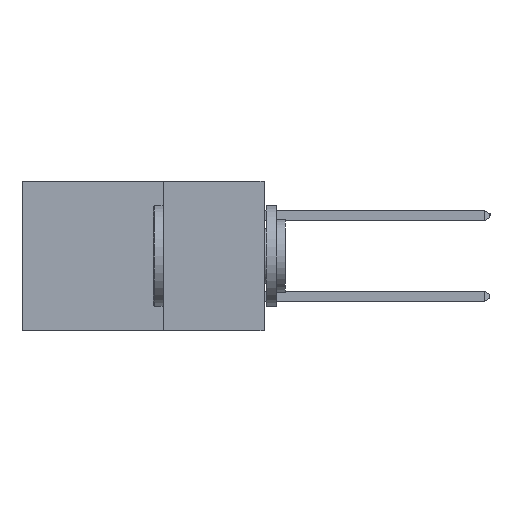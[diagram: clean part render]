
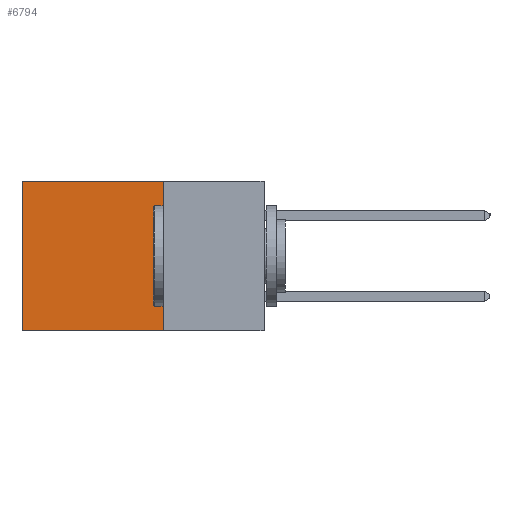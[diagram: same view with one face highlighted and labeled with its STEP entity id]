
A CAD part, left-side view. The second image highlights one B-rep face of the part: STEP entity #6794.
In plain terms, the highlighted planar face has unit normal (-1, 0, 0).
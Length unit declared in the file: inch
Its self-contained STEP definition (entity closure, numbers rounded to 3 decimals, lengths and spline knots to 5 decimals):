
#131 = ORIENTED_EDGE ( 'NONE', *, *, #8737, .F. ) ;
#1723 = VECTOR ( 'NONE', #12689, 39.37008 ) ;
#1924 = EDGE_CURVE ( 'NONE', #6046, #11411, #7034, .T. ) ;
#1972 = LINE ( 'NONE', #4537, #15429 ) ;
#2053 = CARTESIAN_POINT ( 'NONE',  ( 0.2615, 0.25, 0. ) ) ;
#2580 = FACE_OUTER_BOUND ( 'NONE', #4970, .T. ) ;
#3593 = DIRECTION ( 'NONE',  ( 0., 0., -1. ) ) ;
#4027 = VECTOR ( 'NONE', #5826, 39.37008 ) ;
#4089 = EDGE_CURVE ( 'NONE', #14156, #6046, #13797, .T. ) ;
#4537 = CARTESIAN_POINT ( 'NONE',  ( 0.2615, 0.25, -0.37 ) ) ;
#4662 = VERTEX_POINT ( 'NONE', #12997 ) ;
#4766 = CARTESIAN_POINT ( 'NONE',  ( 0.2615, 0.25, 0. ) ) ;
#4970 = EDGE_LOOP ( 'NONE', ( #7160, #16525, #131, #13582 ) ) ;
#5710 = CARTESIAN_POINT ( 'NONE',  ( 0.2615, 0.6, 0. ) ) ;
#5826 = DIRECTION ( 'NONE',  ( 0., 0., -1. ) ) ;
#6046 = VERTEX_POINT ( 'NONE', #5710 ) ;
#6191 = CARTESIAN_POINT ( 'NONE',  ( 0.2615, 0.25, -0.37 ) ) ;
#6794 = ADVANCED_FACE ( 'NONE', ( #2580 ), #12693, .F. ) ;
#7034 = LINE ( 'NONE', #8217, #4027 ) ;
#7160 = ORIENTED_EDGE ( 'NONE', *, *, #1924, .T. ) ;
#8217 = CARTESIAN_POINT ( 'NONE',  ( 0.2615, 0.6, -0.37 ) ) ;
#8737 = EDGE_CURVE ( 'NONE', #14156, #4662, #14152, .T. ) ;
#9319 = VECTOR ( 'NONE', #16523, 39.37008 ) ;
#11200 = CARTESIAN_POINT ( 'NONE',  ( 0.2615, 0.6, -0.37 ) ) ;
#11411 = VERTEX_POINT ( 'NONE', #11200 ) ;
#12074 = AXIS2_PLACEMENT_3D ( 'NONE', #6191, #16629, #3593 ) ;
#12140 = EDGE_CURVE ( 'NONE', #4662, #11411, #1972, .T. ) ;
#12689 = DIRECTION ( 'NONE',  ( 0., 0., -1. ) ) ;
#12693 = PLANE ( 'NONE',  #12074 ) ;
#12854 = CARTESIAN_POINT ( 'NONE',  ( 0.2615, 0.25, -0.37 ) ) ;
#12997 = CARTESIAN_POINT ( 'NONE',  ( 0.2615, 0.25, -0.37 ) ) ;
#13582 = ORIENTED_EDGE ( 'NONE', *, *, #4089, .T. ) ;
#13797 = LINE ( 'NONE', #2053, #9319 ) ;
#14152 = LINE ( 'NONE', #12854, #1723 ) ;
#14156 = VERTEX_POINT ( 'NONE', #4766 ) ;
#15429 = VECTOR ( 'NONE', #16365, 39.37008 ) ;
#16365 = DIRECTION ( 'NONE',  ( 0., 1., 0. ) ) ;
#16523 = DIRECTION ( 'NONE',  ( 0., 1., 0. ) ) ;
#16525 = ORIENTED_EDGE ( 'NONE', *, *, #12140, .F. ) ;
#16629 = DIRECTION ( 'NONE',  ( 1., 0., 0. ) ) ;
